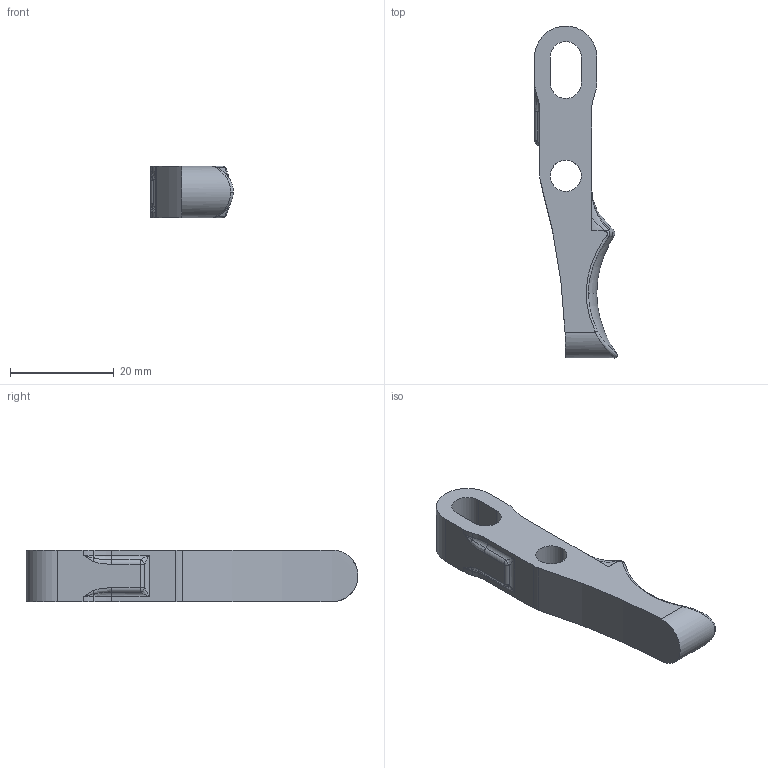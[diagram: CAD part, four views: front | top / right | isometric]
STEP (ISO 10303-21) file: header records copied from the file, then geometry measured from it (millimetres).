
FILE_DESCRIPTION (( 'STEP AP214' ), '1' );
FILE_NAME ('Forward_Trigger.step', '2014-05-14T06:09:35', ( 'WarFairy' ), ( '' ), 'SwSTEP 2.0', 'SolidWorks 2013', '' );
FILE_SCHEMA (( 'AUTOMOTIVE_DESIGN' ));
Length unit declared in the file: inch
Products named in the file (1): Forward_Trigger
Bounding box: 15.97 x 64.06 x 10 mm (x, y, z)
Volume: 5031.3 mm3; surface area: 2869.5 mm2
Topology: 1 solids, 1 shells, 58 faces, 146 edges, 84 vertices
Faces by surface type: cylinder 22, bspline 19, plane 8, torus 7, sphere 2
Entity records: 2980 total; most frequent: CARTESIAN_POINT 1686, ORIENTED_EDGE 280, DIRECTION 240, EDGE_CURVE 140, AXIS2_PLACEMENT_3D 95, VERTEX_POINT 84, EDGE_LOOP 62, ADVANCED_FACE 58
